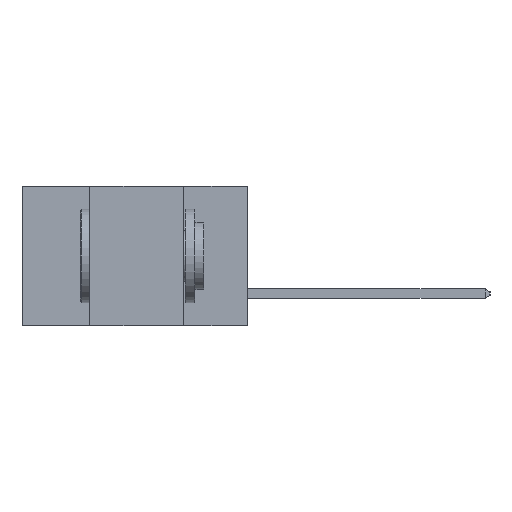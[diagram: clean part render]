
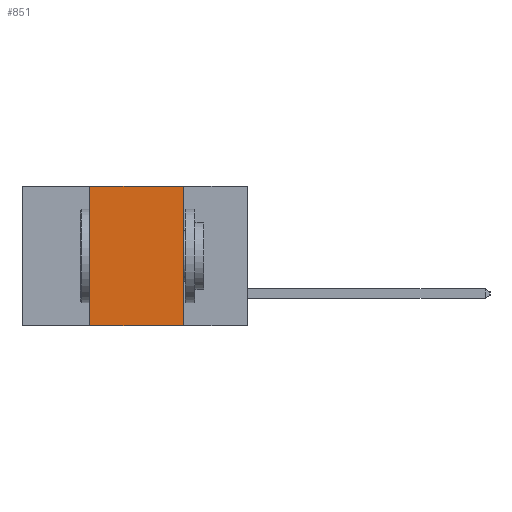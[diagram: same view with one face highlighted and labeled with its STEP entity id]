
A CAD part, left-side view. The second image highlights one B-rep face of the part: STEP entity #851.
In plain terms, the highlighted planar face has unit normal (-1, 0, 0).
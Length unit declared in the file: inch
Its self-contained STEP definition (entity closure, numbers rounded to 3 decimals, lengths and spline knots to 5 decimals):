
#38 = CARTESIAN_POINT ( 'NONE',  ( 0., 0.17, 0. ) ) ;
#127 = VECTOR ( 'NONE', #7701, 39.37008 ) ;
#300 = LINE ( 'NONE', #1098, #12258 ) ;
#519 = DIRECTION ( 'NONE',  ( 0., 0., -1. ) ) ;
#797 = PLANE ( 'NONE',  #10970 ) ;
#851 = ADVANCED_FACE ( 'NONE', ( #7728 ), #797, .F. ) ;
#949 = CARTESIAN_POINT ( 'NONE',  ( 0., 0.17, -0.37 ) ) ;
#1098 = CARTESIAN_POINT ( 'NONE',  ( 0., 0.42, -0.37 ) ) ;
#1099 = VERTEX_POINT ( 'NONE', #10331 ) ;
#1314 = VERTEX_POINT ( 'NONE', #6309 ) ;
#1332 = DIRECTION ( 'NONE',  ( 0., 0., 1. ) ) ;
#1702 = ORIENTED_EDGE ( 'NONE', *, *, #6598, .F. ) ;
#1833 = VERTEX_POINT ( 'NONE', #38 ) ;
#2035 = ORIENTED_EDGE ( 'NONE', *, *, #5276, .F. ) ;
#2270 = VECTOR ( 'NONE', #8154, 39.37008 ) ;
#2394 = VERTEX_POINT ( 'NONE', #7000 ) ;
#2571 = EDGE_LOOP ( 'NONE', ( #1702, #4436, #2035, #7337 ) ) ;
#3257 = EDGE_CURVE ( 'NONE', #1314, #2394, #7540, .T. ) ;
#4436 = ORIENTED_EDGE ( 'NONE', *, *, #5939, .F. ) ;
#5276 = EDGE_CURVE ( 'NONE', #1314, #1099, #300, .T. ) ;
#5690 = VECTOR ( 'NONE', #519, 39.37008 ) ;
#5939 = EDGE_CURVE ( 'NONE', #1099, #1833, #10282, .T. ) ;
#6309 = CARTESIAN_POINT ( 'NONE',  ( 0., 0.42, -0.37 ) ) ;
#6385 = CARTESIAN_POINT ( 'NONE',  ( 0., 0.6, 0. ) ) ;
#6598 = EDGE_CURVE ( 'NONE', #1833, #2394, #8511, .T. ) ;
#7000 = CARTESIAN_POINT ( 'NONE',  ( 0., 0.17, -0.37 ) ) ;
#7337 = ORIENTED_EDGE ( 'NONE', *, *, #3257, .T. ) ;
#7540 = LINE ( 'NONE', #9293, #2270 ) ;
#7701 = DIRECTION ( 'NONE',  ( 0., -1., 0. ) ) ;
#7728 = FACE_OUTER_BOUND ( 'NONE', #2571, .T. ) ;
#7870 = CARTESIAN_POINT ( 'NONE',  ( 0., 0.6, 0. ) ) ;
#8154 = DIRECTION ( 'NONE',  ( 0., -1., 0. ) ) ;
#8511 = LINE ( 'NONE', #949, #5690 ) ;
#9293 = CARTESIAN_POINT ( 'NONE',  ( 0., 0.6, -0.37 ) ) ;
#9984 = DIRECTION ( 'NONE',  ( 1., 0., 0. ) ) ;
#10282 = LINE ( 'NONE', #6385, #127 ) ;
#10331 = CARTESIAN_POINT ( 'NONE',  ( 0., 0.42, 0. ) ) ;
#10970 = AXIS2_PLACEMENT_3D ( 'NONE', #7870, #9984, #12420 ) ;
#12258 = VECTOR ( 'NONE', #1332, 39.37008 ) ;
#12420 = DIRECTION ( 'NONE',  ( 0., 0., -1. ) ) ;
